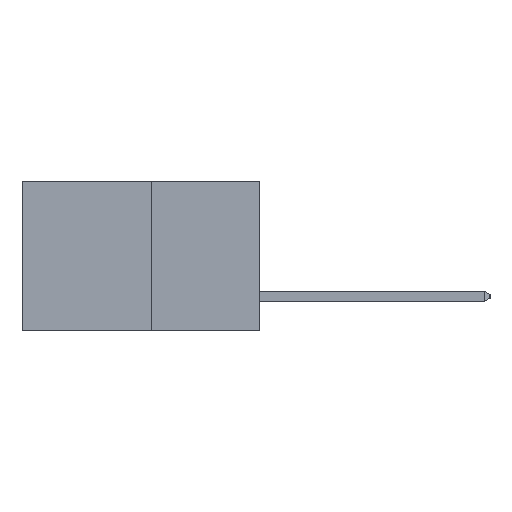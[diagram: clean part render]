
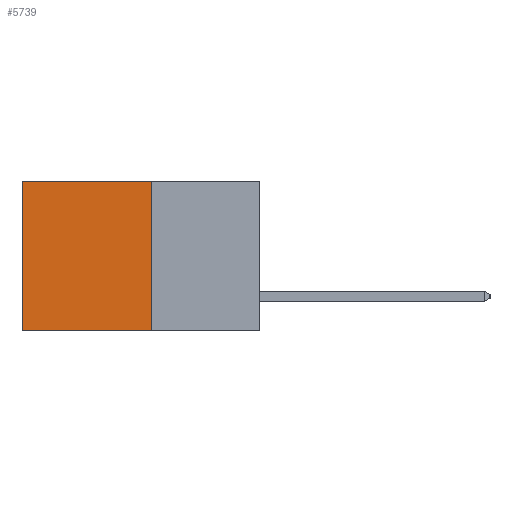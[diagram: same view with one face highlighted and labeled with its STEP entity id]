
A CAD part, left-side view. The second image highlights one B-rep face of the part: STEP entity #5739.
In plain terms, the highlighted planar face has unit normal (-1, 0, 0).
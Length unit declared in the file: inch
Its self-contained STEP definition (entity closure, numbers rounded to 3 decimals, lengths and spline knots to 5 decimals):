
#464 = VECTOR ( 'NONE', #5278, 39.37008 ) ;
#610 = ORIENTED_EDGE ( 'NONE', *, *, #4608, .F. ) ;
#669 = ORIENTED_EDGE ( 'NONE', *, *, #2618, .F. ) ;
#671 = AXIS2_PLACEMENT_3D ( 'NONE', #1377, #985, #867 ) ;
#867 = DIRECTION ( 'NONE',  ( 0., 0., -1. ) ) ;
#903 = LINE ( 'NONE', #3238, #4258 ) ;
#922 = CARTESIAN_POINT ( 'NONE',  ( 0.277, 0.27, 0. ) ) ;
#929 = CARTESIAN_POINT ( 'NONE',  ( 0.277, 0.59, 0. ) ) ;
#985 = DIRECTION ( 'NONE',  ( 1., 0., 0. ) ) ;
#1097 = VERTEX_POINT ( 'NONE', #922 ) ;
#1373 = DIRECTION ( 'NONE',  ( 0., 0., -1. ) ) ;
#1377 = CARTESIAN_POINT ( 'NONE',  ( 0.277, 0.27, -0.37 ) ) ;
#1534 = VERTEX_POINT ( 'NONE', #7511 ) ;
#1602 = LINE ( 'NONE', #7985, #2989 ) ;
#1920 = DIRECTION ( 'NONE',  ( 0., 1., 0. ) ) ;
#2100 = EDGE_CURVE ( 'NONE', #6647, #1534, #903, .T. ) ;
#2610 = VERTEX_POINT ( 'NONE', #6843 ) ;
#2618 = EDGE_CURVE ( 'NONE', #2610, #1534, #1602, .T. ) ;
#2819 = ORIENTED_EDGE ( 'NONE', *, *, #3269, .T. ) ;
#2989 = VECTOR ( 'NONE', #1920, 39.37008 ) ;
#3238 = CARTESIAN_POINT ( 'NONE',  ( 0.277, 0.59, -0.37 ) ) ;
#3269 = EDGE_CURVE ( 'NONE', #1097, #6647, #6933, .T. ) ;
#3621 = VECTOR ( 'NONE', #6035, 39.37008 ) ;
#4258 = VECTOR ( 'NONE', #1373, 39.37008 ) ;
#4390 = EDGE_LOOP ( 'NONE', ( #7114, #669, #610, #2819 ) ) ;
#4608 = EDGE_CURVE ( 'NONE', #1097, #2610, #5708, .T. ) ;
#5278 = DIRECTION ( 'NONE',  ( 0., 1., 0. ) ) ;
#5297 = PLANE ( 'NONE',  #671 ) ;
#5463 = CARTESIAN_POINT ( 'NONE',  ( 0.277, 0.27, -0.37 ) ) ;
#5603 = FACE_OUTER_BOUND ( 'NONE', #4390, .T. ) ;
#5708 = LINE ( 'NONE', #5463, #3621 ) ;
#5739 = ADVANCED_FACE ( 'NONE', ( #5603 ), #5297, .F. ) ;
#6035 = DIRECTION ( 'NONE',  ( 0., 0., -1. ) ) ;
#6647 = VERTEX_POINT ( 'NONE', #929 ) ;
#6843 = CARTESIAN_POINT ( 'NONE',  ( 0.277, 0.27, -0.37 ) ) ;
#6933 = LINE ( 'NONE', #6993, #464 ) ;
#6993 = CARTESIAN_POINT ( 'NONE',  ( 0.277, 0.27, 0. ) ) ;
#7114 = ORIENTED_EDGE ( 'NONE', *, *, #2100, .T. ) ;
#7511 = CARTESIAN_POINT ( 'NONE',  ( 0.277, 0.59, -0.37 ) ) ;
#7985 = CARTESIAN_POINT ( 'NONE',  ( 0.277, 0.27, -0.37 ) ) ;
